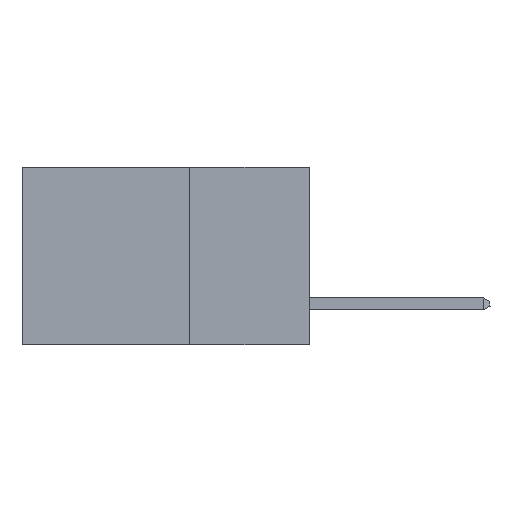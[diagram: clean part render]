
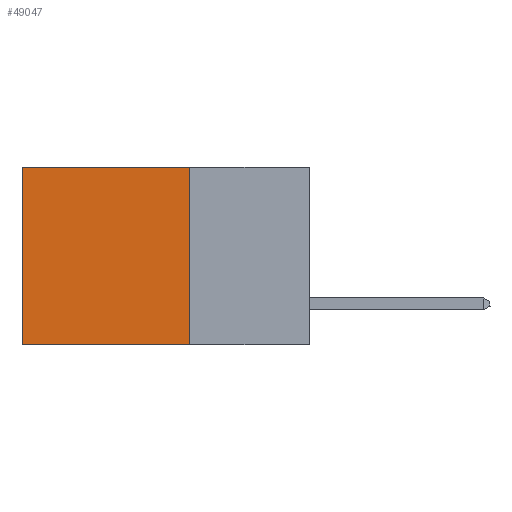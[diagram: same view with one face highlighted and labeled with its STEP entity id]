
A CAD part, left-side view. The second image highlights one B-rep face of the part: STEP entity #49047.
In plain terms, the highlighted planar face has unit normal (-1, 0, 0).
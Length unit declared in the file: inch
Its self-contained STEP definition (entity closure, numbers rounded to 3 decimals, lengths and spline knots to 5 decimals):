
#75 = VECTOR ( 'NONE', #178, 39.37008 ) ;
#178 = DIRECTION ( 'NONE',  ( 0., 1., 0. ) ) ;
#401 = PLANE ( 'NONE',  #13102 ) ;
#4174 = CARTESIAN_POINT ( 'NONE',  ( 0.2875, 0.25, 0. ) ) ;
#4450 = ORIENTED_EDGE ( 'NONE', *, *, #10604, .F. ) ;
#6477 = EDGE_CURVE ( 'NONE', #24291, #31719, #8071, .T. ) ;
#6992 = VERTEX_POINT ( 'NONE', #38672 ) ;
#7333 = LINE ( 'NONE', #28524, #47739 ) ;
#8071 = LINE ( 'NONE', #39403, #75 ) ;
#10029 = CARTESIAN_POINT ( 'NONE',  ( 0.2875, 0.25, 0. ) ) ;
#10408 = LINE ( 'NONE', #10029, #19003 ) ;
#10604 = EDGE_CURVE ( 'NONE', #24291, #6992, #10408, .T. ) ;
#11580 = EDGE_CURVE ( 'NONE', #6992, #18109, #7333, .T. ) ;
#13102 = AXIS2_PLACEMENT_3D ( 'NONE', #4174, #35022, #31597 ) ;
#13959 = FACE_OUTER_BOUND ( 'NONE', #21098, .T. ) ;
#18109 = VERTEX_POINT ( 'NONE', #24505 ) ;
#19003 = VECTOR ( 'NONE', #41360, 39.37008 ) ;
#19675 = ORIENTED_EDGE ( 'NONE', *, *, #11580, .F. ) ;
#20949 = VECTOR ( 'NONE', #42307, 39.37008 ) ;
#21098 = EDGE_LOOP ( 'NONE', ( #40019, #19675, #4450, #40227 ) ) ;
#24291 = VERTEX_POINT ( 'NONE', #33896 ) ;
#24505 = CARTESIAN_POINT ( 'NONE',  ( 0.2875, 0.6, -0.37 ) ) ;
#28071 = EDGE_CURVE ( 'NONE', #31719, #18109, #40535, .T. ) ;
#28524 = CARTESIAN_POINT ( 'NONE',  ( 0.2875, 0.25, -0.37 ) ) ;
#31597 = DIRECTION ( 'NONE',  ( 0., 0., -1. ) ) ;
#31719 = VERTEX_POINT ( 'NONE', #44412 ) ;
#33896 = CARTESIAN_POINT ( 'NONE',  ( 0.2875, 0.25, 0. ) ) ;
#33947 = CARTESIAN_POINT ( 'NONE',  ( 0.2875, 0.6, 0. ) ) ;
#35022 = DIRECTION ( 'NONE',  ( 1., 0., 0. ) ) ;
#38672 = CARTESIAN_POINT ( 'NONE',  ( 0.2875, 0.25, -0.37 ) ) ;
#39403 = CARTESIAN_POINT ( 'NONE',  ( 0.2875, 0.25, 0. ) ) ;
#40019 = ORIENTED_EDGE ( 'NONE', *, *, #28071, .T. ) ;
#40227 = ORIENTED_EDGE ( 'NONE', *, *, #6477, .T. ) ;
#40467 = DIRECTION ( 'NONE',  ( 0., 1., 0. ) ) ;
#40535 = LINE ( 'NONE', #33947, #20949 ) ;
#41360 = DIRECTION ( 'NONE',  ( 0., 0., -1. ) ) ;
#42307 = DIRECTION ( 'NONE',  ( 0., 0., -1. ) ) ;
#44412 = CARTESIAN_POINT ( 'NONE',  ( 0.2875, 0.6, 0. ) ) ;
#47739 = VECTOR ( 'NONE', #40467, 39.37008 ) ;
#49047 = ADVANCED_FACE ( 'NONE', ( #13959 ), #401, .F. ) ;
